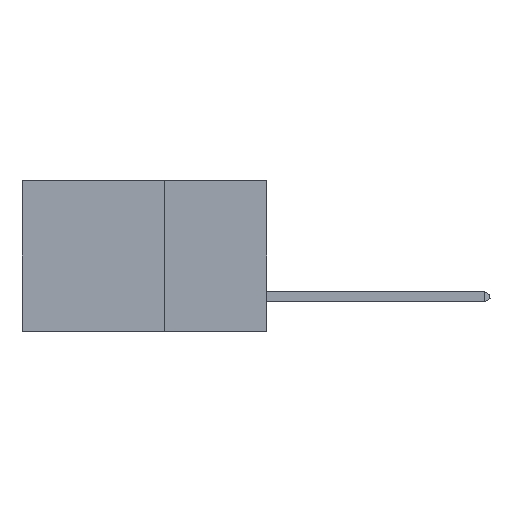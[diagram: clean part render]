
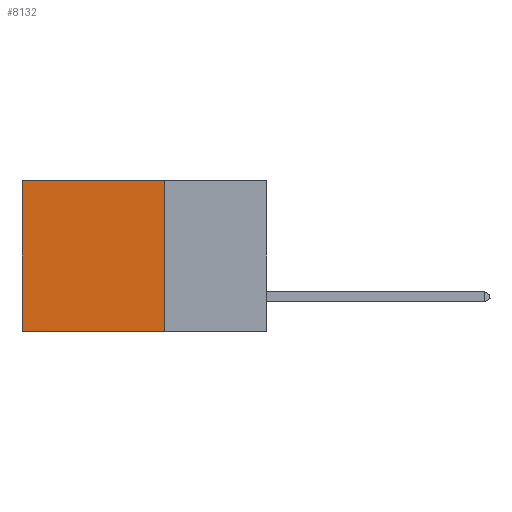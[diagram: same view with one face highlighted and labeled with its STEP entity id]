
A CAD part, left-side view. The second image highlights one B-rep face of the part: STEP entity #8132.
In plain terms, the highlighted planar face has unit normal (-1, 0, 0).
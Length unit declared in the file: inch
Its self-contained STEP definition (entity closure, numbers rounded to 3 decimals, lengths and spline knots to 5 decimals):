
#586 = ORIENTED_EDGE ( 'NONE', *, *, #23474, .T. ) ;
#957 = CARTESIAN_POINT ( 'NONE',  ( 0.2875, 0.25, 0. ) ) ;
#1102 = VECTOR ( 'NONE', #13017, 39.37008 ) ;
#1870 = LINE ( 'NONE', #957, #4593 ) ;
#4067 = EDGE_CURVE ( 'NONE', #16605, #13494, #1870, .T. ) ;
#4593 = VECTOR ( 'NONE', #6847, 39.37008 ) ;
#4893 = PLANE ( 'NONE',  #18482 ) ;
#5472 = EDGE_LOOP ( 'NONE', ( #586, #15275, #14210, #12282 ) ) ;
#6280 = LINE ( 'NONE', #24571, #1102 ) ;
#6847 = DIRECTION ( 'NONE',  ( 0., 1., 0. ) ) ;
#6980 = CARTESIAN_POINT ( 'NONE',  ( 0.2875, 0.6, -0.37 ) ) ;
#8132 = ADVANCED_FACE ( 'NONE', ( #24963 ), #4893, .F. ) ;
#8749 = DIRECTION ( 'NONE',  ( 1., 0., 0. ) ) ;
#8871 = CARTESIAN_POINT ( 'NONE',  ( 0.2875, 0.25, -0.37 ) ) ;
#9924 = CARTESIAN_POINT ( 'NONE',  ( 0.2875, 0.6, 0. ) ) ;
#10492 = VECTOR ( 'NONE', #17437, 39.37008 ) ;
#10840 = VERTEX_POINT ( 'NONE', #6980 ) ;
#11417 = EDGE_CURVE ( 'NONE', #16605, #17220, #6280, .T. ) ;
#12282 = ORIENTED_EDGE ( 'NONE', *, *, #4067, .T. ) ;
#12785 = DIRECTION ( 'NONE',  ( 0., 1., 0. ) ) ;
#12859 = EDGE_CURVE ( 'NONE', #17220, #10840, #21543, .T. ) ;
#13017 = DIRECTION ( 'NONE',  ( 0., 0., -1. ) ) ;
#13494 = VERTEX_POINT ( 'NONE', #22415 ) ;
#13552 = LINE ( 'NONE', #9924, #10492 ) ;
#14210 = ORIENTED_EDGE ( 'NONE', *, *, #11417, .F. ) ;
#15275 = ORIENTED_EDGE ( 'NONE', *, *, #12859, .F. ) ;
#16592 = CARTESIAN_POINT ( 'NONE',  ( 0.2875, 0.25, 0. ) ) ;
#16605 = VERTEX_POINT ( 'NONE', #25133 ) ;
#17204 = CARTESIAN_POINT ( 'NONE',  ( 0.2875, 0.25, -0.37 ) ) ;
#17220 = VERTEX_POINT ( 'NONE', #17204 ) ;
#17437 = DIRECTION ( 'NONE',  ( 0., 0., -1. ) ) ;
#18482 = AXIS2_PLACEMENT_3D ( 'NONE', #16592, #8749, #18552 ) ;
#18552 = DIRECTION ( 'NONE',  ( 0., 0., -1. ) ) ;
#19371 = VECTOR ( 'NONE', #12785, 39.37008 ) ;
#21543 = LINE ( 'NONE', #8871, #19371 ) ;
#22415 = CARTESIAN_POINT ( 'NONE',  ( 0.2875, 0.6, 0. ) ) ;
#23474 = EDGE_CURVE ( 'NONE', #13494, #10840, #13552, .T. ) ;
#24571 = CARTESIAN_POINT ( 'NONE',  ( 0.2875, 0.25, 0. ) ) ;
#24963 = FACE_OUTER_BOUND ( 'NONE', #5472, .T. ) ;
#25133 = CARTESIAN_POINT ( 'NONE',  ( 0.2875, 0.25, 0. ) ) ;
